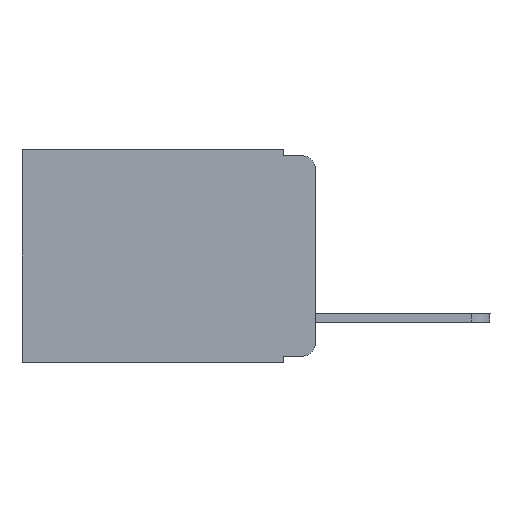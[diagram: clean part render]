
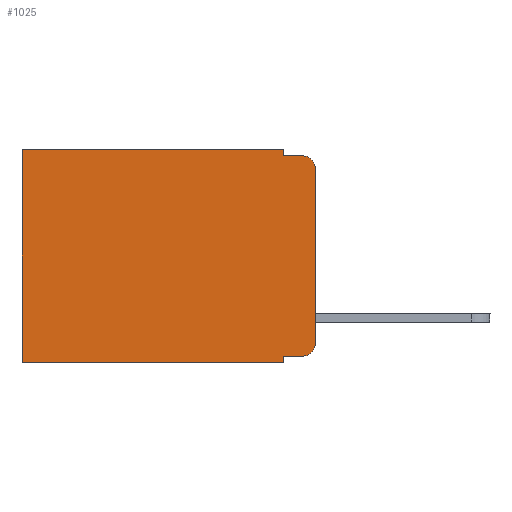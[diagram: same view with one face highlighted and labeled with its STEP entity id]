
A CAD part, left-side view. The second image highlights one B-rep face of the part: STEP entity #1025.
In plain terms, the highlighted planar face has unit normal (-1, 0, 0).
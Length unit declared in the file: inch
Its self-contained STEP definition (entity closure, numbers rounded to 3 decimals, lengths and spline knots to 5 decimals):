
#169 = CARTESIAN_POINT ( 'NONE',  ( 0.298, 0.051, 0. ) ) ;
#229 = DIRECTION ( 'NONE',  ( 0., 0., -1. ) ) ;
#231 = ORIENTED_EDGE ( 'NONE', *, *, #15842, .F. ) ;
#482 = ORIENTED_EDGE ( 'NONE', *, *, #13772, .F. ) ;
#562 = DIRECTION ( 'NONE',  ( 1., 0., 0. ) ) ;
#604 = ORIENTED_EDGE ( 'NONE', *, *, #18400, .F. ) ;
#750 = CARTESIAN_POINT ( 'NONE',  ( 0.298, 0.473, 0. ) ) ;
#1025 = ADVANCED_FACE ( 'NONE', ( #21944 ), #21829, .F. ) ;
#1112 = VERTEX_POINT ( 'NONE', #17012 ) ;
#1440 = LINE ( 'NONE', #20939, #14452 ) ;
#1501 = CARTESIAN_POINT ( 'NONE',  ( 0.298, 0.02, -0.313 ) ) ;
#1866 = CARTESIAN_POINT ( 'NONE',  ( 0.298, 0., 0. ) ) ;
#1869 = VECTOR ( 'NONE', #12256, 39.37008 ) ;
#1987 = VERTEX_POINT ( 'NONE', #2942 ) ;
#2764 = CARTESIAN_POINT ( 'NONE',  ( 0.298, 0.051, -0.01 ) ) ;
#2942 = CARTESIAN_POINT ( 'NONE',  ( 0.298, 0.02, -0.333 ) ) ;
#3188 = ORIENTED_EDGE ( 'NONE', *, *, #14992, .T. ) ;
#3413 = CARTESIAN_POINT ( 'NONE',  ( 0.298, 0.051, -0.333 ) ) ;
#3576 = EDGE_LOOP ( 'NONE', ( #604, #5255, #231, #482, #14275, #14311, #21619, #21975, #3188, #12920 ) ) ;
#3628 = LINE ( 'NONE', #21603, #7853 ) ;
#3660 = CARTESIAN_POINT ( 'NONE',  ( 0.298, 0.051, -0.333 ) ) ;
#3800 = CIRCLE ( 'NONE', #15809, 0.02 ) ;
#4554 = DIRECTION ( 'NONE',  ( 0., 0., -1. ) ) ;
#4867 = VECTOR ( 'NONE', #19152, 39.37008 ) ;
#5054 = LINE ( 'NONE', #6821, #4867 ) ;
#5255 = ORIENTED_EDGE ( 'NONE', *, *, #17379, .T. ) ;
#5274 = LINE ( 'NONE', #1866, #10569 ) ;
#5429 = VERTEX_POINT ( 'NONE', #2764 ) ;
#5739 = VERTEX_POINT ( 'NONE', #750 ) ;
#5963 = CARTESIAN_POINT ( 'NONE',  ( 0.298, 0., 0. ) ) ;
#6821 = CARTESIAN_POINT ( 'NONE',  ( 0.298, 0.051, -0.01 ) ) ;
#6833 = DIRECTION ( 'NONE',  ( 0., -1., 0. ) ) ;
#7851 = VECTOR ( 'NONE', #6833, 39.37008 ) ;
#7853 = VECTOR ( 'NONE', #18068, 39.37008 ) ;
#9219 = CARTESIAN_POINT ( 'NONE',  ( 0.298, 0., -0.313 ) ) ;
#9902 = DIRECTION ( 'NONE',  ( 0., 0., -1. ) ) ;
#10569 = VECTOR ( 'NONE', #229, 39.37008 ) ;
#10962 = DIRECTION ( 'NONE',  ( 0., 1., 0. ) ) ;
#11938 = CARTESIAN_POINT ( 'NONE',  ( 0.298, 0.02, -0.03 ) ) ;
#11994 = CARTESIAN_POINT ( 'NONE',  ( 0.298, 0.051, 0. ) ) ;
#12108 = LINE ( 'NONE', #3413, #7851 ) ;
#12256 = DIRECTION ( 'NONE',  ( 0., 1., 0. ) ) ;
#12920 = ORIENTED_EDGE ( 'NONE', *, *, #21089, .T. ) ;
#13016 = CARTESIAN_POINT ( 'NONE',  ( 0.298, 0., -0.03 ) ) ;
#13716 = DIRECTION ( 'NONE',  ( 0., 0., -1. ) ) ;
#13772 = EDGE_CURVE ( 'NONE', #18114, #5429, #3628, .T. ) ;
#13913 = CARTESIAN_POINT ( 'NONE',  ( 0.298, 0.051, -0.343 ) ) ;
#14275 = ORIENTED_EDGE ( 'NONE', *, *, #19219, .T. ) ;
#14311 = ORIENTED_EDGE ( 'NONE', *, *, #21880, .T. ) ;
#14452 = VECTOR ( 'NONE', #9902, 39.37008 ) ;
#14783 = VECTOR ( 'NONE', #10962, 39.37008 ) ;
#14860 = EDGE_CURVE ( 'NONE', #15033, #19162, #15204, .T. ) ;
#14992 = EDGE_CURVE ( 'NONE', #15033, #1987, #12108, .T. ) ;
#15033 = VERTEX_POINT ( 'NONE', #3660 ) ;
#15204 = LINE ( 'NONE', #11994, #19840 ) ;
#15259 = AXIS2_PLACEMENT_3D ( 'NONE', #5963, #562, #18410 ) ;
#15264 = DIRECTION ( 'NONE',  ( -1., 0., 0. ) ) ;
#15544 = AXIS2_PLACEMENT_3D ( 'NONE', #1501, #17256, #13716 ) ;
#15770 = EDGE_CURVE ( 'NONE', #19162, #23147, #19547, .T. ) ;
#15809 = AXIS2_PLACEMENT_3D ( 'NONE', #11938, #15264, #4554 ) ;
#15842 = EDGE_CURVE ( 'NONE', #5429, #1112, #5054, .T. ) ;
#15920 = CARTESIAN_POINT ( 'NONE',  ( 0.298, 0., 0. ) ) ;
#17012 = CARTESIAN_POINT ( 'NONE',  ( 0.298, 0.02, -0.01 ) ) ;
#17256 = DIRECTION ( 'NONE',  ( -1., 0., 0. ) ) ;
#17297 = VERTEX_POINT ( 'NONE', #13016 ) ;
#17379 = EDGE_CURVE ( 'NONE', #17297, #1112, #3800, .T. ) ;
#17673 = LINE ( 'NONE', #15920, #14783 ) ;
#18068 = DIRECTION ( 'NONE',  ( 0., 0., -1. ) ) ;
#18114 = VERTEX_POINT ( 'NONE', #169 ) ;
#18383 = CARTESIAN_POINT ( 'NONE',  ( 0.298, 0.473, -0.343 ) ) ;
#18400 = EDGE_CURVE ( 'NONE', #17297, #20320, #5274, .T. ) ;
#18410 = DIRECTION ( 'NONE',  ( 0., 0., -1. ) ) ;
#18943 = DIRECTION ( 'NONE',  ( 0., 0., -1. ) ) ;
#19152 = DIRECTION ( 'NONE',  ( 0., -1., 0. ) ) ;
#19162 = VERTEX_POINT ( 'NONE', #13913 ) ;
#19219 = EDGE_CURVE ( 'NONE', #18114, #5739, #17673, .T. ) ;
#19547 = LINE ( 'NONE', #23074, #1869 ) ;
#19840 = VECTOR ( 'NONE', #18943, 39.37008 ) ;
#20320 = VERTEX_POINT ( 'NONE', #9219 ) ;
#20939 = CARTESIAN_POINT ( 'NONE',  ( 0.298, 0.473, 0. ) ) ;
#21089 = EDGE_CURVE ( 'NONE', #1987, #20320, #22304, .T. ) ;
#21603 = CARTESIAN_POINT ( 'NONE',  ( 0.298, 0.051, 0. ) ) ;
#21619 = ORIENTED_EDGE ( 'NONE', *, *, #15770, .F. ) ;
#21829 = PLANE ( 'NONE',  #15259 ) ;
#21880 = EDGE_CURVE ( 'NONE', #5739, #23147, #1440, .T. ) ;
#21944 = FACE_OUTER_BOUND ( 'NONE', #3576, .T. ) ;
#21975 = ORIENTED_EDGE ( 'NONE', *, *, #14860, .F. ) ;
#22304 = CIRCLE ( 'NONE', #15544, 0.02 ) ;
#23074 = CARTESIAN_POINT ( 'NONE',  ( 0.298, 0., -0.343 ) ) ;
#23147 = VERTEX_POINT ( 'NONE', #18383 ) ;
